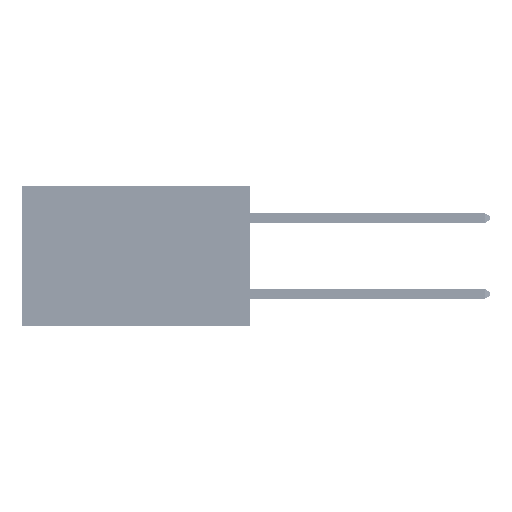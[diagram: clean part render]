
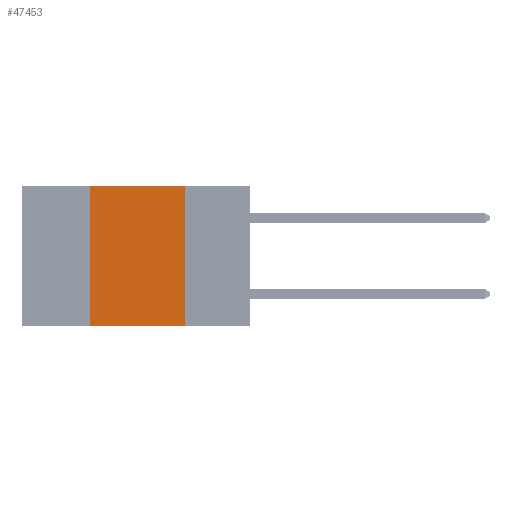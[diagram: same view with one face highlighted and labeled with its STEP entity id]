
A CAD part, left-side view. The second image highlights one B-rep face of the part: STEP entity #47453.
In plain terms, the highlighted planar face has unit normal (-1, 0, 0).
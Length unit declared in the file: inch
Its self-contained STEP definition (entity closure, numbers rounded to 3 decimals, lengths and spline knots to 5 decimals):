
#370 = CARTESIAN_POINT ( 'NONE',  ( 0., 0.17, 0. ) ) ;
#5112 = ORIENTED_EDGE ( 'NONE', *, *, #17985, .F. ) ;
#6511 = VERTEX_POINT ( 'NONE', #18275 ) ;
#8579 = CARTESIAN_POINT ( 'NONE',  ( 0., 0.6, 0. ) ) ;
#9612 = EDGE_LOOP ( 'NONE', ( #24170, #5112, #43762, #10165 ) ) ;
#9641 = DIRECTION ( 'NONE',  ( 0., 0., -1. ) ) ;
#9775 = LINE ( 'NONE', #25427, #23218 ) ;
#10007 = LINE ( 'NONE', #21737, #21549 ) ;
#10143 = VECTOR ( 'NONE', #9641, 39.37008 ) ;
#10165 = ORIENTED_EDGE ( 'NONE', *, *, #36089, .T. ) ;
#14821 = EDGE_CURVE ( 'NONE', #17145, #22584, #31878, .T. ) ;
#16187 = VECTOR ( 'NONE', #26636, 39.37008 ) ;
#17145 = VERTEX_POINT ( 'NONE', #370 ) ;
#17484 = LINE ( 'NONE', #39178, #16187 ) ;
#17985 = EDGE_CURVE ( 'NONE', #19543, #17145, #17484, .T. ) ;
#18275 = CARTESIAN_POINT ( 'NONE',  ( 0., 0.42, -0.37 ) ) ;
#19543 = VERTEX_POINT ( 'NONE', #23468 ) ;
#21089 = PLANE ( 'NONE',  #42364 ) ;
#21141 = DIRECTION ( 'NONE',  ( 0., 0., 1. ) ) ;
#21209 = DIRECTION ( 'NONE',  ( 0., -1., 0. ) ) ;
#21549 = VECTOR ( 'NONE', #21209, 39.37008 ) ;
#21737 = CARTESIAN_POINT ( 'NONE',  ( 0., 0.6, -0.37 ) ) ;
#22584 = VERTEX_POINT ( 'NONE', #51648 ) ;
#23218 = VECTOR ( 'NONE', #21141, 39.37008 ) ;
#23468 = CARTESIAN_POINT ( 'NONE',  ( 0., 0.42, 0. ) ) ;
#24170 = ORIENTED_EDGE ( 'NONE', *, *, #14821, .F. ) ;
#24840 = DIRECTION ( 'NONE',  ( 1., 0., 0. ) ) ;
#25014 = DIRECTION ( 'NONE',  ( 0., 0., -1. ) ) ;
#25427 = CARTESIAN_POINT ( 'NONE',  ( 0., 0.42, 0. ) ) ;
#26636 = DIRECTION ( 'NONE',  ( 0., -1., 0. ) ) ;
#29129 = CARTESIAN_POINT ( 'NONE',  ( 0., 0.17, 0. ) ) ;
#31878 = LINE ( 'NONE', #29129, #10143 ) ;
#36089 = EDGE_CURVE ( 'NONE', #6511, #22584, #10007, .T. ) ;
#39178 = CARTESIAN_POINT ( 'NONE',  ( 0., 0.6, 0. ) ) ;
#40179 = EDGE_CURVE ( 'NONE', #6511, #19543, #9775, .T. ) ;
#42364 = AXIS2_PLACEMENT_3D ( 'NONE', #8579, #24840, #25014 ) ;
#43762 = ORIENTED_EDGE ( 'NONE', *, *, #40179, .F. ) ;
#43970 = FACE_OUTER_BOUND ( 'NONE', #9612, .T. ) ;
#47453 = ADVANCED_FACE ( 'NONE', ( #43970 ), #21089, .F. ) ;
#51648 = CARTESIAN_POINT ( 'NONE',  ( 0., 0.17, -0.37 ) ) ;
